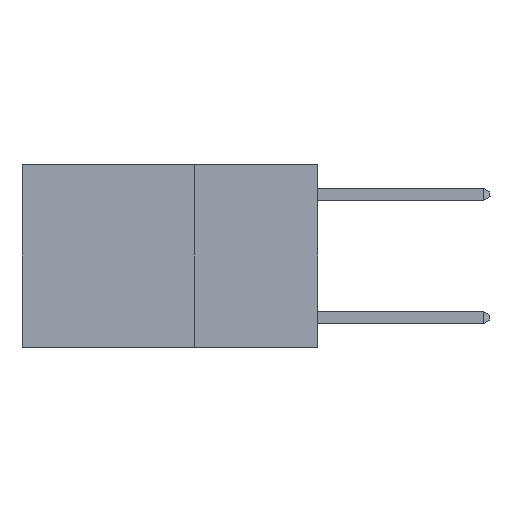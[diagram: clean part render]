
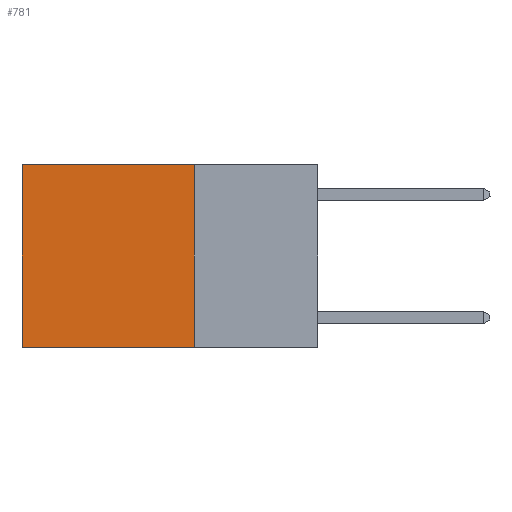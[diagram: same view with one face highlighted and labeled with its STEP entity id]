
A CAD part, left-side view. The second image highlights one B-rep face of the part: STEP entity #781.
In plain terms, the highlighted planar face has unit normal (-1, 0, 0).
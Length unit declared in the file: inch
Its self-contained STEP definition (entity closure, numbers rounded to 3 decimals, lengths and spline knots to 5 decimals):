
#781 = ADVANCED_FACE ( 'NONE', ( #14126 ), #7482, .F. ) ;
#2290 = DIRECTION ( 'NONE',  ( 0., 0., -1. ) ) ;
#2350 = CARTESIAN_POINT ( 'NONE',  ( 0.2625, 0.25, 0. ) ) ;
#2771 = VECTOR ( 'NONE', #5702, 39.37008 ) ;
#2887 = EDGE_CURVE ( 'NONE', #10107, #7689, #15069, .T. ) ;
#2925 = VECTOR ( 'NONE', #9830, 39.37008 ) ;
#3719 = DIRECTION ( 'NONE',  ( 0., 0., -1. ) ) ;
#3764 = LINE ( 'NONE', #9780, #2925 ) ;
#4317 = LINE ( 'NONE', #10986, #10604 ) ;
#5593 = CARTESIAN_POINT ( 'NONE',  ( 0.2625, 0.25, 0. ) ) ;
#5702 = DIRECTION ( 'NONE',  ( 0., 1., 0. ) ) ;
#5736 = EDGE_CURVE ( 'NONE', #7689, #7760, #6322, .T. ) ;
#5746 = VERTEX_POINT ( 'NONE', #14168 ) ;
#6322 = LINE ( 'NONE', #12988, #2771 ) ;
#6359 = CARTESIAN_POINT ( 'NONE',  ( 0.2625, 0.25, 0. ) ) ;
#7269 = ORIENTED_EDGE ( 'NONE', *, *, #16033, .T. ) ;
#7316 = ORIENTED_EDGE ( 'NONE', *, *, #5736, .F. ) ;
#7355 = ORIENTED_EDGE ( 'NONE', *, *, #2887, .F. ) ;
#7377 = ORIENTED_EDGE ( 'NONE', *, *, #11937, .T. ) ;
#7482 = PLANE ( 'NONE',  #13210 ) ;
#7645 = EDGE_LOOP ( 'NONE', ( #7269, #7316, #7355, #7377 ) ) ;
#7689 = VERTEX_POINT ( 'NONE', #15309 ) ;
#7760 = VERTEX_POINT ( 'NONE', #11861 ) ;
#9780 = CARTESIAN_POINT ( 'NONE',  ( 0.2625, 0.25, 0. ) ) ;
#9830 = DIRECTION ( 'NONE',  ( 0., 1., 0. ) ) ;
#10107 = VERTEX_POINT ( 'NONE', #6359 ) ;
#10604 = VECTOR ( 'NONE', #15735, 39.37008 ) ;
#10986 = CARTESIAN_POINT ( 'NONE',  ( 0.2625, 0.6, 0. ) ) ;
#11861 = CARTESIAN_POINT ( 'NONE',  ( 0.2625, 0.6, -0.37 ) ) ;
#11928 = VECTOR ( 'NONE', #2290, 39.37008 ) ;
#11937 = EDGE_CURVE ( 'NONE', #10107, #5746, #3764, .T. ) ;
#12988 = CARTESIAN_POINT ( 'NONE',  ( 0.2625, 0.25, -0.37 ) ) ;
#13210 = AXIS2_PLACEMENT_3D ( 'NONE', #5593, #15633, #3719 ) ;
#14126 = FACE_OUTER_BOUND ( 'NONE', #7645, .T. ) ;
#14168 = CARTESIAN_POINT ( 'NONE',  ( 0.2625, 0.6, 0. ) ) ;
#15069 = LINE ( 'NONE', #2350, #11928 ) ;
#15309 = CARTESIAN_POINT ( 'NONE',  ( 0.2625, 0.25, -0.37 ) ) ;
#15633 = DIRECTION ( 'NONE',  ( 1., 0., 0. ) ) ;
#15735 = DIRECTION ( 'NONE',  ( 0., 0., -1. ) ) ;
#16033 = EDGE_CURVE ( 'NONE', #5746, #7760, #4317, .T. ) ;
